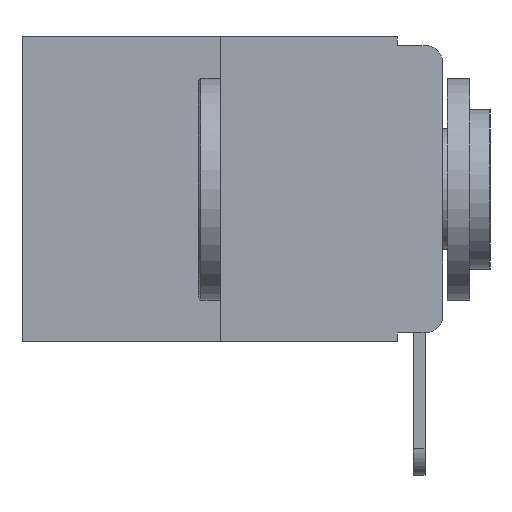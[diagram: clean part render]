
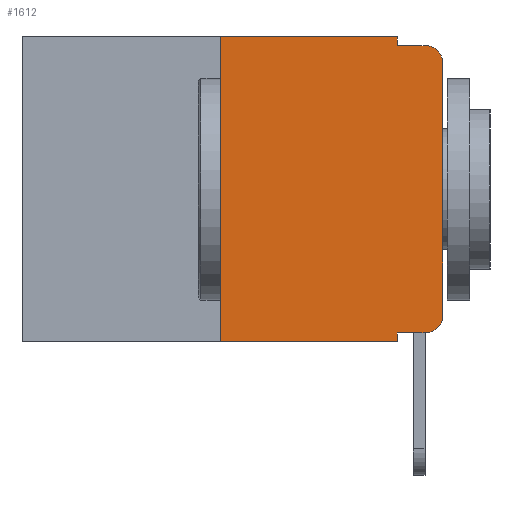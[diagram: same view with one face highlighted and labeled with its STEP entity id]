
A CAD part, left-side view. The second image highlights one B-rep face of the part: STEP entity #1612.
In plain terms, the highlighted planar face has unit normal (-1, 0, 0).
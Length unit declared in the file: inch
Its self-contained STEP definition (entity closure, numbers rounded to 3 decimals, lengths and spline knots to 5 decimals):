
#255 = CARTESIAN_POINT ( 'NONE',  ( 0., 0.25, -0.343 ) ) ;
#502 = VERTEX_POINT ( 'NONE', #15609 ) ;
#561 = CIRCLE ( 'NONE', #13369, 0.02 ) ;
#784 = VERTEX_POINT ( 'NONE', #8257 ) ;
#993 = LINE ( 'NONE', #3593, #20672 ) ;
#1497 = DIRECTION ( 'NONE',  ( 0., 0., 1. ) ) ;
#1612 = ADVANCED_FACE ( 'NONE', ( #3178 ), #20364, .F. ) ;
#1968 = DIRECTION ( 'NONE',  ( -1., 0., 0. ) ) ;
#2276 = EDGE_LOOP ( 'NONE', ( #12133, #19409, #12433, #17374, #20509, #5076, #17886, #13881, #18906, #14816 ) ) ;
#2883 = DIRECTION ( 'NONE',  ( 0., 0., -1. ) ) ;
#3100 = CARTESIAN_POINT ( 'NONE',  ( 0., 0.473, 0. ) ) ;
#3178 = FACE_OUTER_BOUND ( 'NONE', #2276, .T. ) ;
#3462 = CARTESIAN_POINT ( 'NONE',  ( 0., 0.25, 0. ) ) ;
#3592 = VERTEX_POINT ( 'NONE', #5933 ) ;
#3593 = CARTESIAN_POINT ( 'NONE',  ( 0., 0.051, -0.333 ) ) ;
#4504 = VERTEX_POINT ( 'NONE', #16601 ) ;
#4747 = EDGE_CURVE ( 'NONE', #784, #3592, #993, .T. ) ;
#4839 = DIRECTION ( 'NONE',  ( 1., 0., 0. ) ) ;
#5076 = ORIENTED_EDGE ( 'NONE', *, *, #16953, .F. ) ;
#5598 = VERTEX_POINT ( 'NONE', #255 ) ;
#5774 = CIRCLE ( 'NONE', #17097, 0.02 ) ;
#5933 = CARTESIAN_POINT ( 'NONE',  ( 0., 0.02, -0.333 ) ) ;
#6563 = VERTEX_POINT ( 'NONE', #17186 ) ;
#6578 = LINE ( 'NONE', #10515, #12453 ) ;
#7083 = LINE ( 'NONE', #18684, #8706 ) ;
#7353 = EDGE_CURVE ( 'NONE', #5598, #502, #12869, .T. ) ;
#7829 = CARTESIAN_POINT ( 'NONE',  ( 0., 0.02, -0.313 ) ) ;
#7877 = EDGE_CURVE ( 'NONE', #784, #502, #22512, .T. ) ;
#7896 = VERTEX_POINT ( 'NONE', #17457 ) ;
#7963 = VERTEX_POINT ( 'NONE', #18056 ) ;
#8053 = VERTEX_POINT ( 'NONE', #13184 ) ;
#8257 = CARTESIAN_POINT ( 'NONE',  ( 0., 0.051, -0.333 ) ) ;
#8365 = CARTESIAN_POINT ( 'NONE',  ( 0., 0.02, -0.03 ) ) ;
#8706 = VECTOR ( 'NONE', #15675, 39.37008 ) ;
#8764 = DIRECTION ( 'NONE',  ( 0., 0., 1. ) ) ;
#8769 = EDGE_CURVE ( 'NONE', #3592, #7896, #561, .T. ) ;
#8817 = DIRECTION ( 'NONE',  ( 0., 0., -1. ) ) ;
#8829 = DIRECTION ( 'NONE',  ( 0., 0., -1. ) ) ;
#8916 = EDGE_CURVE ( 'NONE', #7963, #8053, #7083, .T. ) ;
#9411 = CARTESIAN_POINT ( 'NONE',  ( 0., 0., -0.03 ) ) ;
#10239 = VECTOR ( 'NONE', #8817, 39.37008 ) ;
#10324 = CARTESIAN_POINT ( 'NONE',  ( 0., 0., 0. ) ) ;
#10515 = CARTESIAN_POINT ( 'NONE',  ( 0., 0.051, -0.01 ) ) ;
#10587 = CARTESIAN_POINT ( 'NONE',  ( 0., 0.051, 0. ) ) ;
#12027 = VECTOR ( 'NONE', #1497, 39.37008 ) ;
#12117 = EDGE_CURVE ( 'NONE', #14122, #6563, #5774, .T. ) ;
#12133 = ORIENTED_EDGE ( 'NONE', *, *, #12720, .T. ) ;
#12433 = ORIENTED_EDGE ( 'NONE', *, *, #17552, .F. ) ;
#12453 = VECTOR ( 'NONE', #14103, 39.37008 ) ;
#12720 = EDGE_CURVE ( 'NONE', #7896, #14122, #21336, .T. ) ;
#12869 = LINE ( 'NONE', #16345, #19993 ) ;
#13184 = CARTESIAN_POINT ( 'NONE',  ( 0., 0.051, 0. ) ) ;
#13322 = DIRECTION ( 'NONE',  ( -1., 0., 0. ) ) ;
#13369 = AXIS2_PLACEMENT_3D ( 'NONE', #7829, #13322, #2883 ) ;
#13881 = ORIENTED_EDGE ( 'NONE', *, *, #7877, .F. ) ;
#13961 = DIRECTION ( 'NONE',  ( 0., -1., 0. ) ) ;
#14103 = DIRECTION ( 'NONE',  ( 0., -1., 0. ) ) ;
#14122 = VERTEX_POINT ( 'NONE', #9411 ) ;
#14700 = EDGE_CURVE ( 'NONE', #8053, #4504, #15987, .T. ) ;
#14816 = ORIENTED_EDGE ( 'NONE', *, *, #8769, .T. ) ;
#15609 = CARTESIAN_POINT ( 'NONE',  ( 0., 0.051, -0.343 ) ) ;
#15675 = DIRECTION ( 'NONE',  ( 0., -1., 0. ) ) ;
#15761 = DIRECTION ( 'NONE',  ( 0., 0., -1. ) ) ;
#15987 = LINE ( 'NONE', #19533, #10239 ) ;
#16345 = CARTESIAN_POINT ( 'NONE',  ( 0., 0.473, -0.343 ) ) ;
#16601 = CARTESIAN_POINT ( 'NONE',  ( 0., 0.051, -0.01 ) ) ;
#16644 = DIRECTION ( 'NONE',  ( 0., -1., 0. ) ) ;
#16788 = VECTOR ( 'NONE', #8829, 39.37008 ) ;
#16953 = EDGE_CURVE ( 'NONE', #5598, #7963, #21666, .T. ) ;
#17097 = AXIS2_PLACEMENT_3D ( 'NONE', #8365, #1968, #15761 ) ;
#17186 = CARTESIAN_POINT ( 'NONE',  ( 0., 0.02, -0.01 ) ) ;
#17374 = ORIENTED_EDGE ( 'NONE', *, *, #14700, .F. ) ;
#17457 = CARTESIAN_POINT ( 'NONE',  ( 0., 0., -0.313 ) ) ;
#17552 = EDGE_CURVE ( 'NONE', #4504, #6563, #6578, .T. ) ;
#17886 = ORIENTED_EDGE ( 'NONE', *, *, #7353, .T. ) ;
#18056 = CARTESIAN_POINT ( 'NONE',  ( 0., 0.25, 0. ) ) ;
#18529 = AXIS2_PLACEMENT_3D ( 'NONE', #3100, #4839, #22045 ) ;
#18684 = CARTESIAN_POINT ( 'NONE',  ( 0., 0.473, 0. ) ) ;
#18906 = ORIENTED_EDGE ( 'NONE', *, *, #4747, .T. ) ;
#19409 = ORIENTED_EDGE ( 'NONE', *, *, #12117, .T. ) ;
#19533 = CARTESIAN_POINT ( 'NONE',  ( 0., 0.051, 0. ) ) ;
#19993 = VECTOR ( 'NONE', #16644, 39.37008 ) ;
#20364 = PLANE ( 'NONE',  #18529 ) ;
#20509 = ORIENTED_EDGE ( 'NONE', *, *, #8916, .F. ) ;
#20672 = VECTOR ( 'NONE', #13961, 39.37008 ) ;
#21123 = VECTOR ( 'NONE', #8764, 39.37008 ) ;
#21336 = LINE ( 'NONE', #10324, #12027 ) ;
#21666 = LINE ( 'NONE', #3462, #21123 ) ;
#22045 = DIRECTION ( 'NONE',  ( 0., 0., -1. ) ) ;
#22512 = LINE ( 'NONE', #10587, #16788 ) ;
